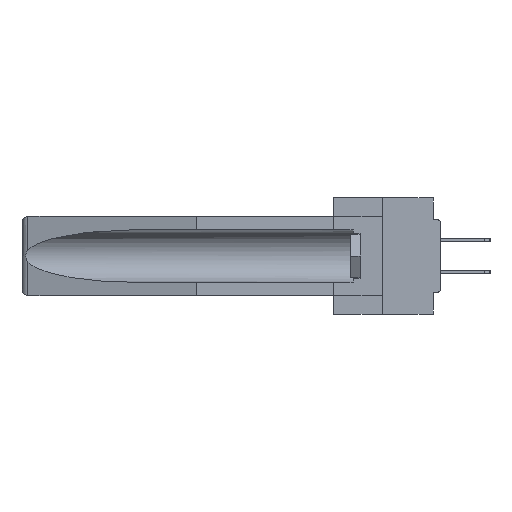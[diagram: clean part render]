
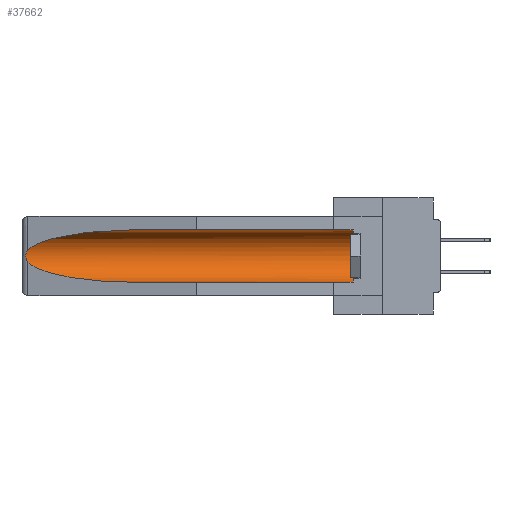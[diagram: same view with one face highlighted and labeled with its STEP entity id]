
A CAD part, left-side view. The second image highlights one B-rep face of the part: STEP entity #37662.
In plain terms, the highlighted cylindrical face has radius 2.857 mm (diameter 5.715 mm), a partial arc.
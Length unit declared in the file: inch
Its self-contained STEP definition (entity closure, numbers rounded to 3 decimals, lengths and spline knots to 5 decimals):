
#150 = CARTESIAN_POINT ( 'NONE',  ( 0.26597, 1.5296, -0.19026 ) ) ;
#204 = LINE ( 'NONE', #11689, #26652 ) ;
#358 = EDGE_CURVE ( 'NONE', #25721, #6188, #29089, .T. ) ;
#434 = CARTESIAN_POINT ( 'NONE',  ( 0.155, 1.07973, -0.284 ) ) ;
#1371 = ORIENTED_EDGE ( 'NONE', *, *, #9356, .T. ) ;
#3105 = CARTESIAN_POINT ( 'NONE',  ( 0.26537, 1.52718, -0.19328 ) ) ;
#5351 = CARTESIAN_POINT ( 'NONE',  ( 0.21114, 1.30732, -0.059 ) ) ;
#5768 = CARTESIAN_POINT ( 'NONE',  ( 0.155, 0.126, -0.059 ) ) ;
#6188 = VERTEX_POINT ( 'NONE', #35137 ) ;
#6878 = CARTESIAN_POINT ( 'NONE',  ( 0.26537, 1.52718, -0.14972 ) ) ;
#7240 = EDGE_CURVE ( 'NONE', #24134, #20846, #42693, .T. ) ;
#8561 = DIRECTION ( 'NONE',  ( 0., -1., 0. ) ) ;
#8675 = CARTESIAN_POINT ( 'NONE',  ( 0.155, 0.126, -0.284 ) ) ;
#9147 =( BOUNDED_CURVE ( )  B_SPLINE_CURVE ( 3, ( #21842, #5351, #29761, #39476 ),
 .UNSPECIFIED., .F., .F. ) 
 B_SPLINE_CURVE_WITH_KNOTS ( ( 4, 4 ),
 ( 4.71239, 6.08839 ),
 .UNSPECIFIED. ) 
 CURVE ( )  GEOMETRIC_REPRESENTATION_ITEM ( )  RATIONAL_B_SPLINE_CURVE ( ( 1., 0.848, 0.848, 1. ) ) 
 REPRESENTATION_ITEM ( '' )  );
#9356 = EDGE_CURVE ( 'NONE', #15385, #25721, #9147, .T. ) ;
#9379 = ORIENTED_EDGE ( 'NONE', *, *, #7240, .T. ) ;
#9425 = DIRECTION ( 'NONE',  ( 0., 1., 0. ) ) ;
#10044 = CARTESIAN_POINT ( 'NONE',  ( 0.26537, 1.52718, -0.19328 ) ) ;
#10195 = CARTESIAN_POINT ( 'NONE',  ( 0.2675, 1.53308, -0.17534 ) ) ;
#10549 = CARTESIAN_POINT ( 'NONE',  ( 0.155, 1.07973, -0.284 ) ) ;
#10574 = CARTESIAN_POINT ( 'NONE',  ( 0.155, -0.30754, -0.059 ) ) ;
#11689 = CARTESIAN_POINT ( 'NONE',  ( 0.155, -0.30754, -0.284 ) ) ;
#13794 = DIRECTION ( 'NONE',  ( 0., 1., 0. ) ) ;
#15385 = VERTEX_POINT ( 'NONE', #36933 ) ;
#15932 = CARTESIAN_POINT ( 'NONE',  ( 0.155, -0.30754, -0.1715 ) ) ;
#17008 = ORIENTED_EDGE ( 'NONE', *, *, #18921, .T. ) ;
#17021 = CARTESIAN_POINT ( 'NONE',  ( 0.26597, 1.52961, -0.15275 ) ) ;
#17585 = ORIENTED_EDGE ( 'NONE', *, *, #358, .T. ) ;
#18921 = EDGE_CURVE ( 'NONE', #20846, #15385, #24662, .T. ) ;
#19251 = ORIENTED_EDGE ( 'NONE', *, *, #35250, .F. ) ;
#19409 = DIRECTION ( 'NONE',  ( 0., 0., 1. ) ) ;
#20009 = CARTESIAN_POINT ( 'NONE',  ( 0.26655, 1.53094, -0.18657 ) ) ;
#20163 = CARTESIAN_POINT ( 'NONE',  ( 0.26654, 1.53092, -0.15636 ) ) ;
#20429 = CARTESIAN_POINT ( 'NONE',  ( 0.21114, 1.30732, -0.284 ) ) ;
#20846 = VERTEX_POINT ( 'NONE', #5768 ) ;
#21842 = CARTESIAN_POINT ( 'NONE',  ( 0.155, 1.07973, -0.059 ) ) ;
#22848 = VERTEX_POINT ( 'NONE', #10549 ) ;
#23058 = CARTESIAN_POINT ( 'NONE',  ( 0.2673, 1.5327, -0.16383 ) ) ;
#23341 = FACE_OUTER_BOUND ( 'NONE', #32936, .T. ) ;
#23514 = CARTESIAN_POINT ( 'NONE',  ( 0.26537, 1.52718, -0.14972 ) ) ;
#24134 = VERTEX_POINT ( 'NONE', #8675 ) ;
#24662 = LINE ( 'NONE', #10574, #32918 ) ;
#25043 = CARTESIAN_POINT ( 'NONE',  ( 0.155, 0.126, -0.1715 ) ) ;
#25673 = CARTESIAN_POINT ( 'NONE',  ( 0.25451, 1.48313, -0.24835 ) ) ;
#25721 = VERTEX_POINT ( 'NONE', #6878 ) ;
#26652 = VECTOR ( 'NONE', #32043, 39.37008 ) ;
#29089 = B_SPLINE_CURVE_WITH_KNOTS ( 'NONE', 3,
 ( #23514, #17021, #20163, #23058, #29835, #10195, #29687, #20009, #150, #10044 ),
 .UNSPECIFIED., .F., .F.,
 ( 4, 2, 2, 2, 4 ),
 ( 0., 0.00029, 0.00058, 0.00087, 0.00117 ),
 .UNSPECIFIED. ) ;
#29687 = CARTESIAN_POINT ( 'NONE',  ( 0.2673, 1.53269, -0.17917 ) ) ;
#29761 = CARTESIAN_POINT ( 'NONE',  ( 0.25451, 1.48313, -0.09465 ) ) ;
#29835 = CARTESIAN_POINT ( 'NONE',  ( 0.2675, 1.53308, -0.16763 ) ) ;
#31691 = DIRECTION ( 'NONE',  ( 0., 0., 1. ) ) ;
#32043 = DIRECTION ( 'NONE',  ( 0., 1., 0. ) ) ;
#32918 = VECTOR ( 'NONE', #13794, 39.37008 ) ;
#32936 = EDGE_LOOP ( 'NONE', ( #1371, #17585, #37305, #19251, #9379, #17008 ) ) ;
#34242 = CYLINDRICAL_SURFACE ( 'NONE', #38221, 0.1125 ) ;
#35137 = CARTESIAN_POINT ( 'NONE',  ( 0.26537, 1.52718, -0.19328 ) ) ;
#35250 = EDGE_CURVE ( 'NONE', #24134, #22848, #204, .T. ) ;
#35410 = EDGE_CURVE ( 'NONE', #6188, #22848, #36835, .T. ) ;
#36835 =( BOUNDED_CURVE ( )  B_SPLINE_CURVE ( 3, ( #3105, #25673, #20429, #434 ),
 .UNSPECIFIED., .F., .T. ) 
 B_SPLINE_CURVE_WITH_KNOTS ( ( 4, 4 ),
 ( 0.1948, 1.5708 ),
 .UNSPECIFIED. ) 
 CURVE ( )  GEOMETRIC_REPRESENTATION_ITEM ( )  RATIONAL_B_SPLINE_CURVE ( ( 1., 0.848, 0.848, 1. ) ) 
 REPRESENTATION_ITEM ( '' )  );
#36933 = CARTESIAN_POINT ( 'NONE',  ( 0.155, 1.07973, -0.059 ) ) ;
#37080 = AXIS2_PLACEMENT_3D ( 'NONE', #25043, #8561, #31691 ) ;
#37305 = ORIENTED_EDGE ( 'NONE', *, *, #35410, .T. ) ;
#37662 = ADVANCED_FACE ( 'NONE', ( #23341 ), #34242, .F. ) ;
#38221 = AXIS2_PLACEMENT_3D ( 'NONE', #15932, #9425, #19409 ) ;
#39476 = CARTESIAN_POINT ( 'NONE',  ( 0.26537, 1.52718, -0.14972 ) ) ;
#42693 = CIRCLE ( 'NONE', #37080, 0.1125 ) ;
